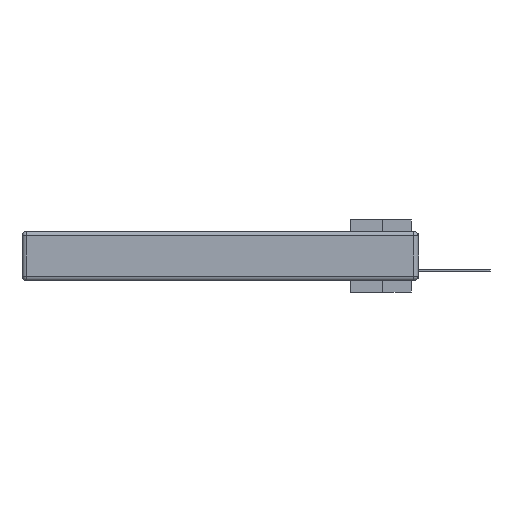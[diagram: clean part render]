
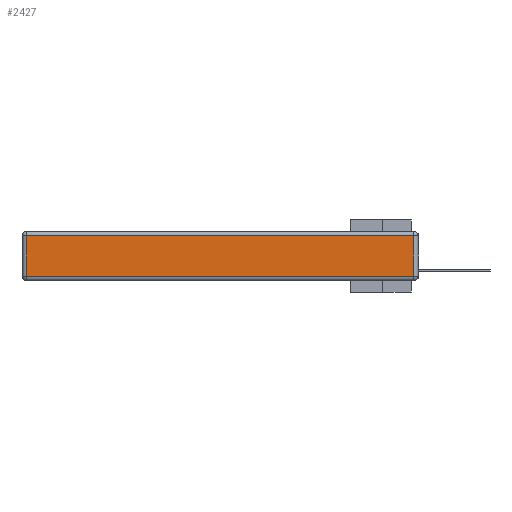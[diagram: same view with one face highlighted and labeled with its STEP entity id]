
A CAD part, left-side view. The second image highlights one B-rep face of the part: STEP entity #2427.
In plain terms, the highlighted planar face has unit normal (-1, 0, 0).
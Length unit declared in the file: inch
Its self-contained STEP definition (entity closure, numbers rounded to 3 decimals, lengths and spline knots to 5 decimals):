
#931 = DIRECTION ( 'NONE',  ( 0., -1., 0. ) ) ;
#1427 = CARTESIAN_POINT ( 'NONE',  ( 0., 0., -0.343 ) ) ;
#1922 = DIRECTION ( 'NONE',  ( -1., 0., 0. ) ) ;
#2093 = DIRECTION ( 'NONE',  ( 0., 0., 1. ) ) ;
#2427 = ADVANCED_FACE ( 'NONE', ( #4292 ), #24731, .T. ) ;
#3366 = CARTESIAN_POINT ( 'NONE',  ( 0., 2.72, -0.03 ) ) ;
#4152 = CARTESIAN_POINT ( 'NONE',  ( 0., 0.03, -0.313 ) ) ;
#4292 = FACE_OUTER_BOUND ( 'NONE', #18356, .T. ) ;
#5027 = DIRECTION ( 'NONE',  ( 0., 1., 0. ) ) ;
#5101 = VERTEX_POINT ( 'NONE', #21900 ) ;
#6479 = ORIENTED_EDGE ( 'NONE', *, *, #28176, .T. ) ;
#6948 = LINE ( 'NONE', #20249, #7584 ) ;
#7584 = VECTOR ( 'NONE', #12233, 39.37008 ) ;
#8408 = LINE ( 'NONE', #18794, #17529 ) ;
#12233 = DIRECTION ( 'NONE',  ( 0., 0., -1. ) ) ;
#13792 = VECTOR ( 'NONE', #931, 39.37008 ) ;
#15199 = ORIENTED_EDGE ( 'NONE', *, *, #31639, .T. ) ;
#15981 = CARTESIAN_POINT ( 'NONE',  ( 0., 0.03, -0.03 ) ) ;
#16011 = VERTEX_POINT ( 'NONE', #15981 ) ;
#16095 = CARTESIAN_POINT ( 'NONE',  ( 0., 0.03, -0.343 ) ) ;
#17529 = VECTOR ( 'NONE', #5027, 39.37008 ) ;
#18356 = EDGE_LOOP ( 'NONE', ( #6479, #23043, #15199, #31037 ) ) ;
#18794 = CARTESIAN_POINT ( 'NONE',  ( 0., 2.75, -0.03 ) ) ;
#20249 = CARTESIAN_POINT ( 'NONE',  ( 0., 2.72, -0.343 ) ) ;
#20253 = VECTOR ( 'NONE', #29222, 39.37008 ) ;
#21900 = CARTESIAN_POINT ( 'NONE',  ( 0., 2.72, -0.313 ) ) ;
#22304 = EDGE_CURVE ( 'NONE', #27752, #5101, #6948, .T. ) ;
#23043 = ORIENTED_EDGE ( 'NONE', *, *, #31161, .T. ) ;
#24245 = LINE ( 'NONE', #31561, #13792 ) ;
#24731 = PLANE ( 'NONE',  #27539 ) ;
#26008 = LINE ( 'NONE', #16095, #20253 ) ;
#27539 = AXIS2_PLACEMENT_3D ( 'NONE', #1427, #1922, #2093 ) ;
#27752 = VERTEX_POINT ( 'NONE', #3366 ) ;
#28176 = EDGE_CURVE ( 'NONE', #5101, #32935, #24245, .T. ) ;
#29222 = DIRECTION ( 'NONE',  ( 0., 0., 1. ) ) ;
#31037 = ORIENTED_EDGE ( 'NONE', *, *, #22304, .T. ) ;
#31161 = EDGE_CURVE ( 'NONE', #32935, #16011, #26008, .T. ) ;
#31561 = CARTESIAN_POINT ( 'NONE',  ( 0., 0., -0.313 ) ) ;
#31639 = EDGE_CURVE ( 'NONE', #16011, #27752, #8408, .T. ) ;
#32935 = VERTEX_POINT ( 'NONE', #4152 ) ;
